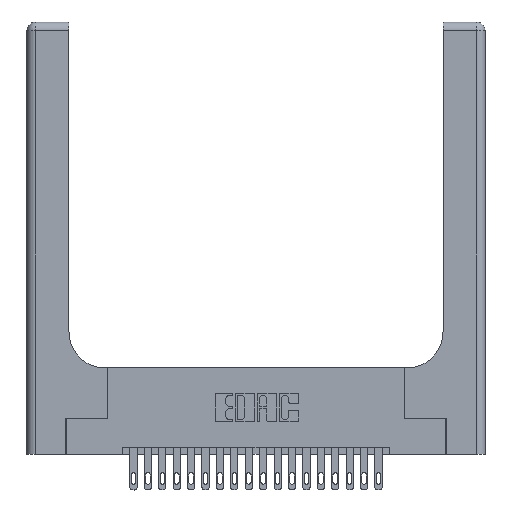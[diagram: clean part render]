
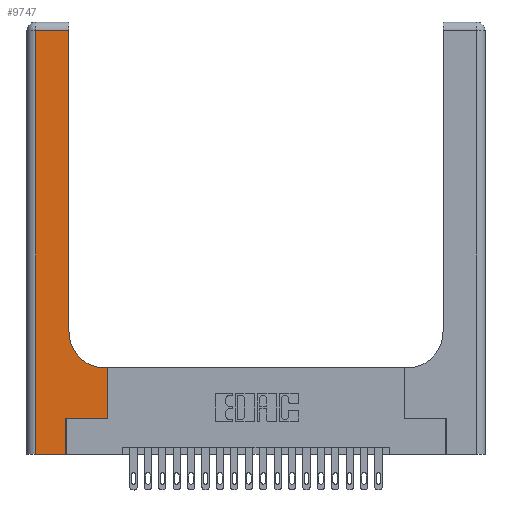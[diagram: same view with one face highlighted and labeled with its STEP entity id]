
A CAD part, top view. The second image highlights one B-rep face of the part: STEP entity #9747.
In plain terms, the highlighted planar face has unit normal (0, 0, 1).
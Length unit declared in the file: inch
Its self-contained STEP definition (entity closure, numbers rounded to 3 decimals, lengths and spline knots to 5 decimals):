
#71 = VECTOR ( 'NONE', #6492, 39.37008 ) ;
#176 = EDGE_CURVE ( 'NONE', #5220, #21076, #3357, .T. ) ;
#543 = DIRECTION ( 'NONE',  ( 0., -1., 0. ) ) ;
#852 = CARTESIAN_POINT ( 'NONE',  ( 0.5585, 0.25, 0.37 ) ) ;
#1139 = AXIS2_PLACEMENT_3D ( 'NONE', #1711, #15615, #8926 ) ;
#1307 = CARTESIAN_POINT ( 'NONE',  ( 0., 2.94, 0.37 ) ) ;
#1711 = CARTESIAN_POINT ( 'NONE',  ( 0.5415, 0.85, 0.37 ) ) ;
#1818 = EDGE_CURVE ( 'NONE', #7413, #5220, #5788, .T. ) ;
#1865 = ORIENTED_EDGE ( 'NONE', *, *, #176, .T. ) ;
#2303 = VERTEX_POINT ( 'NONE', #21651 ) ;
#2354 = LINE ( 'NONE', #852, #6473 ) ;
#2430 = LINE ( 'NONE', #7204, #4894 ) ;
#2487 = EDGE_CURVE ( 'NONE', #6193, #10791, #6073, .T. ) ;
#2714 = EDGE_LOOP ( 'NONE', ( #16933, #18570, #15922, #10643, #1865, #15405, #10942, #15661, #19832 ) ) ;
#3357 = LINE ( 'NONE', #20346, #16674 ) ;
#4033 = VECTOR ( 'NONE', #20260, 39.37008 ) ;
#4054 = DIRECTION ( 'NONE',  ( 0., 1., 0. ) ) ;
#4343 = CARTESIAN_POINT ( 'NONE',  ( 0.2915, 2.94, 0.37 ) ) ;
#4894 = VECTOR ( 'NONE', #17779, 39.37008 ) ;
#5220 = VERTEX_POINT ( 'NONE', #5877 ) ;
#5580 = DIRECTION ( 'NONE',  ( -1., 0., 0. ) ) ;
#5625 = CARTESIAN_POINT ( 'NONE',  ( 0.06, 0., 0.37 ) ) ;
#5692 = EDGE_CURVE ( 'NONE', #2303, #7883, #2354, .T. ) ;
#5788 = LINE ( 'NONE', #12089, #71 ) ;
#5877 = CARTESIAN_POINT ( 'NONE',  ( 0.269, 0., 0.37 ) ) ;
#5883 = CARTESIAN_POINT ( 'NONE',  ( 0.06, 3., 0.37 ) ) ;
#5946 = LINE ( 'NONE', #14910, #4033 ) ;
#6073 = CIRCLE ( 'NONE', #1139, 0.25 ) ;
#6193 = VERTEX_POINT ( 'NONE', #19111 ) ;
#6281 = EDGE_CURVE ( 'NONE', #18366, #12768, #21905, .T. ) ;
#6473 = VECTOR ( 'NONE', #4054, 39.37008 ) ;
#6492 = DIRECTION ( 'NONE',  ( 1., 0., 0. ) ) ;
#7204 = CARTESIAN_POINT ( 'NONE',  ( 0.2915, 3., 0.37 ) ) ;
#7413 = VERTEX_POINT ( 'NONE', #5625 ) ;
#7883 = VERTEX_POINT ( 'NONE', #19868 ) ;
#8926 = DIRECTION ( 'NONE',  ( 1., 0., 0. ) ) ;
#9599 = CARTESIAN_POINT ( 'NONE',  ( 0., 3., 0.37 ) ) ;
#9747 = ADVANCED_FACE ( 'NONE', ( #12287 ), #14893, .F. ) ;
#10356 = LINE ( 'NONE', #5883, #18236 ) ;
#10500 = VECTOR ( 'NONE', #20464, 39.37008 ) ;
#10643 = ORIENTED_EDGE ( 'NONE', *, *, #1818, .T. ) ;
#10791 = VERTEX_POINT ( 'NONE', #12765 ) ;
#10869 = CARTESIAN_POINT ( 'NONE',  ( 0.06, 2.94, 0.37 ) ) ;
#10876 = EDGE_CURVE ( 'NONE', #12768, #7413, #10356, .T. ) ;
#10942 = ORIENTED_EDGE ( 'NONE', *, *, #5692, .T. ) ;
#12089 = CARTESIAN_POINT ( 'NONE',  ( 0., 0., 0.37 ) ) ;
#12287 = FACE_OUTER_BOUND ( 'NONE', #2714, .T. ) ;
#12364 = CARTESIAN_POINT ( 'NONE',  ( 0.269, 0.25, 0.37 ) ) ;
#12765 = CARTESIAN_POINT ( 'NONE',  ( 0.2915, 0.85, 0.37 ) ) ;
#12768 = VERTEX_POINT ( 'NONE', #10869 ) ;
#12843 = VECTOR ( 'NONE', #5580, 39.37008 ) ;
#13007 = DIRECTION ( 'NONE',  ( -1., 0., 0. ) ) ;
#13014 = AXIS2_PLACEMENT_3D ( 'NONE', #9599, #21731, #13007 ) ;
#14321 = EDGE_CURVE ( 'NONE', #7883, #6193, #20217, .T. ) ;
#14893 = PLANE ( 'NONE',  #13014 ) ;
#14910 = CARTESIAN_POINT ( 'NONE',  ( 0.269, 0.25, 0.37 ) ) ;
#15305 = DIRECTION ( 'NONE',  ( 0., 1., 0. ) ) ;
#15405 = ORIENTED_EDGE ( 'NONE', *, *, #17807, .T. ) ;
#15615 = DIRECTION ( 'NONE',  ( 0., 0., -1. ) ) ;
#15661 = ORIENTED_EDGE ( 'NONE', *, *, #14321, .T. ) ;
#15922 = ORIENTED_EDGE ( 'NONE', *, *, #10876, .T. ) ;
#16501 = EDGE_CURVE ( 'NONE', #10791, #18366, #2430, .T. ) ;
#16674 = VECTOR ( 'NONE', #15305, 39.37008 ) ;
#16933 = ORIENTED_EDGE ( 'NONE', *, *, #16501, .T. ) ;
#17779 = DIRECTION ( 'NONE',  ( 0., 1., 0. ) ) ;
#17807 = EDGE_CURVE ( 'NONE', #21076, #2303, #5946, .T. ) ;
#18236 = VECTOR ( 'NONE', #543, 39.37008 ) ;
#18366 = VERTEX_POINT ( 'NONE', #4343 ) ;
#18570 = ORIENTED_EDGE ( 'NONE', *, *, #6281, .T. ) ;
#19111 = CARTESIAN_POINT ( 'NONE',  ( 0.5415, 0.6, 0.37 ) ) ;
#19832 = ORIENTED_EDGE ( 'NONE', *, *, #2487, .T. ) ;
#19868 = CARTESIAN_POINT ( 'NONE',  ( 0.5585, 0.6, 0.37 ) ) ;
#20217 = LINE ( 'NONE', #21351, #12843 ) ;
#20260 = DIRECTION ( 'NONE',  ( 1., 0., 0. ) ) ;
#20346 = CARTESIAN_POINT ( 'NONE',  ( 0.269, 0., 0.37 ) ) ;
#20464 = DIRECTION ( 'NONE',  ( -1., 0., 0. ) ) ;
#21076 = VERTEX_POINT ( 'NONE', #12364 ) ;
#21351 = CARTESIAN_POINT ( 'NONE',  ( 0.2915, 0.6, 0.37 ) ) ;
#21651 = CARTESIAN_POINT ( 'NONE',  ( 0.5585, 0.25, 0.37 ) ) ;
#21731 = DIRECTION ( 'NONE',  ( 0., 0., -1. ) ) ;
#21905 = LINE ( 'NONE', #1307, #10500 ) ;
